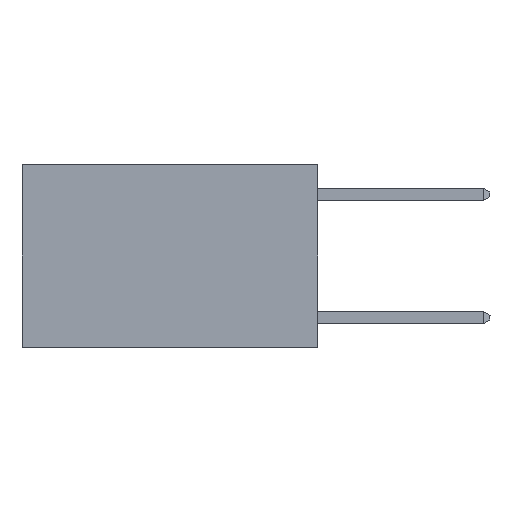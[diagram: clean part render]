
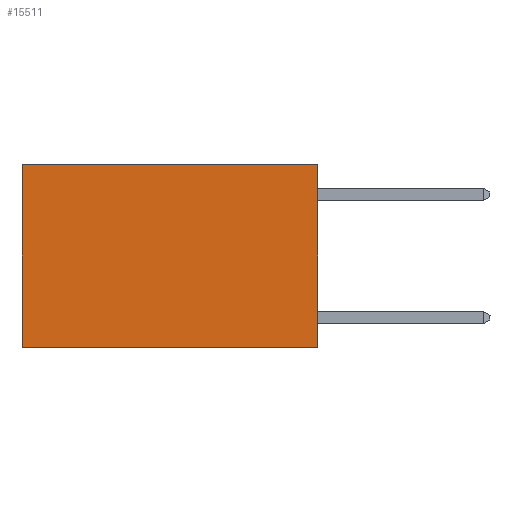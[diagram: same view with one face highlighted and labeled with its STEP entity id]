
A CAD part, left-side view. The second image highlights one B-rep face of the part: STEP entity #15511.
In plain terms, the highlighted planar face has unit normal (-1, 0, 0).
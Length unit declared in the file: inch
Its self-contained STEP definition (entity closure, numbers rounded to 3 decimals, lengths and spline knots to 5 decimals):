
#444 = CARTESIAN_POINT ( 'NONE',  ( 0.2625, 0., 0. ) ) ;
#544 = CARTESIAN_POINT ( 'NONE',  ( 0.2625, 0.6, -0.37 ) ) ;
#1861 = DIRECTION ( 'NONE',  ( 0., 0., -1. ) ) ;
#2241 = ORIENTED_EDGE ( 'NONE', *, *, #17703, .F. ) ;
#2707 = PLANE ( 'NONE',  #14711 ) ;
#3930 = CARTESIAN_POINT ( 'NONE',  ( 0.2625, 0., -0.37 ) ) ;
#4129 = DIRECTION ( 'NONE',  ( 0., 0., -1. ) ) ;
#4642 = EDGE_LOOP ( 'NONE', ( #16850, #7814, #2241, #7173 ) ) ;
#4664 = CARTESIAN_POINT ( 'NONE',  ( 0.2625, 0., 0. ) ) ;
#4985 = CARTESIAN_POINT ( 'NONE',  ( 0.2625, 0.6, 0. ) ) ;
#6837 = VECTOR ( 'NONE', #9202, 39.37008 ) ;
#7173 = ORIENTED_EDGE ( 'NONE', *, *, #15044, .T. ) ;
#7273 = LINE ( 'NONE', #4985, #6837 ) ;
#7387 = VECTOR ( 'NONE', #15703, 39.37008 ) ;
#7494 = DIRECTION ( 'NONE',  ( 0., 1., 0. ) ) ;
#7814 = ORIENTED_EDGE ( 'NONE', *, *, #11457, .F. ) ;
#8271 = FACE_OUTER_BOUND ( 'NONE', #4642, .T. ) ;
#8287 = VERTEX_POINT ( 'NONE', #9164 ) ;
#8808 = VECTOR ( 'NONE', #7494, 39.37008 ) ;
#9164 = CARTESIAN_POINT ( 'NONE',  ( 0.2625, 0.6, 0. ) ) ;
#9202 = DIRECTION ( 'NONE',  ( 0., 0., -1. ) ) ;
#9681 = CARTESIAN_POINT ( 'NONE',  ( 0.2625, 0., 0. ) ) ;
#10212 = EDGE_CURVE ( 'NONE', #8287, #17741, #7273, .T. ) ;
#10487 = LINE ( 'NONE', #4664, #12852 ) ;
#11457 = EDGE_CURVE ( 'NONE', #15996, #17741, #12487, .T. ) ;
#11647 = CARTESIAN_POINT ( 'NONE',  ( 0.2625, 0., 0. ) ) ;
#12435 = DIRECTION ( 'NONE',  ( 1., 0., 0. ) ) ;
#12487 = LINE ( 'NONE', #13009, #8808 ) ;
#12852 = VECTOR ( 'NONE', #1861, 39.37008 ) ;
#13009 = CARTESIAN_POINT ( 'NONE',  ( 0.2625, 0., -0.37 ) ) ;
#14711 = AXIS2_PLACEMENT_3D ( 'NONE', #9681, #12435, #4129 ) ;
#14752 = LINE ( 'NONE', #444, #7387 ) ;
#15044 = EDGE_CURVE ( 'NONE', #15686, #8287, #14752, .T. ) ;
#15511 = ADVANCED_FACE ( 'NONE', ( #8271 ), #2707, .F. ) ;
#15686 = VERTEX_POINT ( 'NONE', #11647 ) ;
#15703 = DIRECTION ( 'NONE',  ( 0., 1., 0. ) ) ;
#15996 = VERTEX_POINT ( 'NONE', #3930 ) ;
#16850 = ORIENTED_EDGE ( 'NONE', *, *, #10212, .T. ) ;
#17703 = EDGE_CURVE ( 'NONE', #15686, #15996, #10487, .T. ) ;
#17741 = VERTEX_POINT ( 'NONE', #544 ) ;
